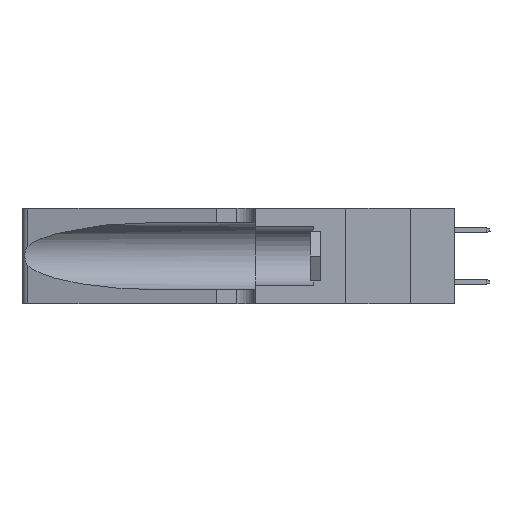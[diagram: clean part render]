
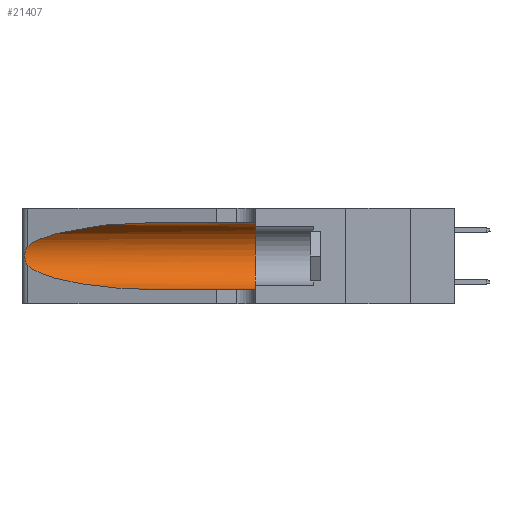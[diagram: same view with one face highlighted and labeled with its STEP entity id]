
A CAD part, left-side view. The second image highlights one B-rep face of the part: STEP entity #21407.
In plain terms, the highlighted cylindrical face has radius 3.308 mm (diameter 6.617 mm), a partial arc.
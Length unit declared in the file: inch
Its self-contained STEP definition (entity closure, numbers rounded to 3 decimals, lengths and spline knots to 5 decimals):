
#1585 = CARTESIAN_POINT ( 'NONE',  ( 0.25639, 1.23186, 0.15144 ) ) ;
#1752 = CARTESIAN_POINT ( 'NONE',  ( 0.25487, 1.22718, 0.22369 ) ) ;
#2560 = EDGE_CURVE ( 'NONE', #12100, #7527, #3603, .T. ) ;
#2877 = VERTEX_POINT ( 'NONE', #25615 ) ;
#3603 = LINE ( 'NONE', #30120, #9734 ) ;
#3942 = CARTESIAN_POINT ( 'NONE',  ( 0.18966, 0.96281, 0.31525 ) ) ;
#4154 = CARTESIAN_POINT ( 'NONE',  ( 0.26017, 1.23833, 0.17102 ) ) ;
#5109 = EDGE_CURVE ( 'NONE', #19245, #19274, #32990, .T. ) ;
#5358 = DIRECTION ( 'NONE',  ( 0., 0., 1. ) ) ;
#6436 = DIRECTION ( 'NONE',  ( 0., 0., -1. ) ) ;
#6448 = ORIENTED_EDGE ( 'NONE', *, *, #7016, .T. ) ;
#6693 = CARTESIAN_POINT ( 'NONE',  ( 0.26075, 1.23896, 0.19203 ) ) ;
#7016 = EDGE_CURVE ( 'NONE', #12100, #2877, #24759, .T. ) ;
#7039 = CARTESIAN_POINT ( 'NONE',  ( 0.25487, 1.22718, 0.14631 ) ) ;
#7132 = ORIENTED_EDGE ( 'NONE', *, *, #25310, .F. ) ;
#7171 = B_SPLINE_CURVE_WITH_KNOTS ( 'NONE', 3,
 ( #1752, #19547, #29497, #29829, #14501, #27277, #6693, #17005, #4154, #12101, #24714, #1585, #13997, #30004 ),
 .UNSPECIFIED., .F., .F.,
 ( 4, 2, 2, 2, 2, 2, 4 ),
 ( 0., 0.00027, 0.00053, 0.00107, 0.0016, 0.00187, 0.00214 ),
 .UNSPECIFIED. ) ;
#7527 = VERTEX_POINT ( 'NONE', #17685 ) ;
#7813 = CARTESIAN_POINT ( 'NONE',  ( 0.1305, 0.35, 0.05475 ) ) ;
#9589 = EDGE_LOOP ( 'NONE', ( #6448, #29951, #14391, #14756, #7132, #25110 ) ) ;
#9734 = VECTOR ( 'NONE', #16476, 39.37008 ) ;
#10240 = AXIS2_PLACEMENT_3D ( 'NONE', #24955, #17083, #6436 ) ;
#10801 = VERTEX_POINT ( 'NONE', #7813 ) ;
#10820 = CARTESIAN_POINT ( 'NONE',  ( 0.1305, 0.72297, 0.05475 ) ) ;
#11772 = EDGE_CURVE ( 'NONE', #2877, #19245, #7171, .T. ) ;
#12100 = VERTEX_POINT ( 'NONE', #17590 ) ;
#12101 = CARTESIAN_POINT ( 'NONE',  ( 0.25856, 1.23593, 0.16098 ) ) ;
#13198 = CIRCLE ( 'NONE', #19668, 0.13025 ) ;
#13515 = CARTESIAN_POINT ( 'NONE',  ( 0.1305, 0.35, 0.185 ) ) ;
#13997 = CARTESIAN_POINT ( 'NONE',  ( 0.25555, 1.22993, 0.14849 ) ) ;
#14391 = ORIENTED_EDGE ( 'NONE', *, *, #5109, .T. ) ;
#14501 = CARTESIAN_POINT ( 'NONE',  ( 0.25854, 1.2359, 0.20912 ) ) ;
#14756 = ORIENTED_EDGE ( 'NONE', *, *, #16178, .T. ) ;
#16178 = EDGE_CURVE ( 'NONE', #19274, #10801, #23955, .T. ) ;
#16301 = CARTESIAN_POINT ( 'NONE',  ( 0.1305, 0.72297, 0.31525 ) ) ;
#16476 = DIRECTION ( 'NONE',  ( 0., -1., 0. ) ) ;
#16923 = VECTOR ( 'NONE', #27324, 39.37008 ) ;
#17005 = CARTESIAN_POINT ( 'NONE',  ( 0.26075, 1.23896, 0.178 ) ) ;
#17083 = DIRECTION ( 'NONE',  ( 0., -1., 0. ) ) ;
#17590 = CARTESIAN_POINT ( 'NONE',  ( 0.1305, 0.72297, 0.31525 ) ) ;
#17685 = CARTESIAN_POINT ( 'NONE',  ( 0.1305, 0.35, 0.31525 ) ) ;
#19245 = VERTEX_POINT ( 'NONE', #7039 ) ;
#19274 = VERTEX_POINT ( 'NONE', #20246 ) ;
#19547 = CARTESIAN_POINT ( 'NONE',  ( 0.25555, 1.22994, 0.2215 ) ) ;
#19668 = AXIS2_PLACEMENT_3D ( 'NONE', #13515, #23759, #5358 ) ;
#20246 = CARTESIAN_POINT ( 'NONE',  ( 0.1305, 0.72297, 0.05475 ) ) ;
#21407 = ADVANCED_FACE ( 'NONE', ( #29576 ), #22133, .F. ) ;
#22133 = CYLINDRICAL_SURFACE ( 'NONE', #10240, 0.13025 ) ;
#22701 = CARTESIAN_POINT ( 'NONE',  ( 0.18966, 0.96281, 0.05475 ) ) ;
#23197 = CARTESIAN_POINT ( 'NONE',  ( 0.25487, 1.22718, 0.14631 ) ) ;
#23759 = DIRECTION ( 'NONE',  ( 0., 1., 0. ) ) ;
#23955 = LINE ( 'NONE', #24124, #16923 ) ;
#24027 = CARTESIAN_POINT ( 'NONE',  ( 0.2373, 1.15595, 0.28018 ) ) ;
#24124 = CARTESIAN_POINT ( 'NONE',  ( 0.1305, 1.61858, 0.05475 ) ) ;
#24714 = CARTESIAN_POINT ( 'NONE',  ( 0.25789, 1.23486, 0.15765 ) ) ;
#24759 =( BOUNDED_CURVE ( )  B_SPLINE_CURVE ( 3, ( #16301, #3942, #24027, #29782 ),
 .UNSPECIFIED., .F., .T. ) 
 B_SPLINE_CURVE_WITH_KNOTS ( ( 4, 4 ),
 ( 1.5708, 2.84003 ),
 .UNSPECIFIED. ) 
 CURVE ( )  GEOMETRIC_REPRESENTATION_ITEM ( )  RATIONAL_B_SPLINE_CURVE ( ( 1., 0.87, 0.87, 1. ) ) 
 REPRESENTATION_ITEM ( '' )  );
#24955 = CARTESIAN_POINT ( 'NONE',  ( 0.1305, 1.61858, 0.185 ) ) ;
#25110 = ORIENTED_EDGE ( 'NONE', *, *, #2560, .F. ) ;
#25210 = CARTESIAN_POINT ( 'NONE',  ( 0.2373, 1.15595, 0.08982 ) ) ;
#25310 = EDGE_CURVE ( 'NONE', #7527, #10801, #13198, .T. ) ;
#25615 = CARTESIAN_POINT ( 'NONE',  ( 0.25487, 1.22718, 0.22369 ) ) ;
#27277 = CARTESIAN_POINT ( 'NONE',  ( 0.26018, 1.23835, 0.19895 ) ) ;
#27324 = DIRECTION ( 'NONE',  ( 0., -1., 0. ) ) ;
#29497 = CARTESIAN_POINT ( 'NONE',  ( 0.25639, 1.23184, 0.21858 ) ) ;
#29576 = FACE_OUTER_BOUND ( 'NONE', #9589, .T. ) ;
#29782 = CARTESIAN_POINT ( 'NONE',  ( 0.25487, 1.22718, 0.22369 ) ) ;
#29829 = CARTESIAN_POINT ( 'NONE',  ( 0.25787, 1.23484, 0.2124 ) ) ;
#29951 = ORIENTED_EDGE ( 'NONE', *, *, #11772, .T. ) ;
#30004 = CARTESIAN_POINT ( 'NONE',  ( 0.25487, 1.22718, 0.14631 ) ) ;
#30120 = CARTESIAN_POINT ( 'NONE',  ( 0.1305, 1.61858, 0.31525 ) ) ;
#32990 =( BOUNDED_CURVE ( )  B_SPLINE_CURVE ( 3, ( #23197, #25210, #22701, #10820 ),
 .UNSPECIFIED., .F., .T. ) 
 B_SPLINE_CURVE_WITH_KNOTS ( ( 4, 4 ),
 ( 3.44316, 4.71239 ),
 .UNSPECIFIED. ) 
 CURVE ( )  GEOMETRIC_REPRESENTATION_ITEM ( )  RATIONAL_B_SPLINE_CURVE ( ( 1., 0.87, 0.87, 1. ) ) 
 REPRESENTATION_ITEM ( '' )  );
